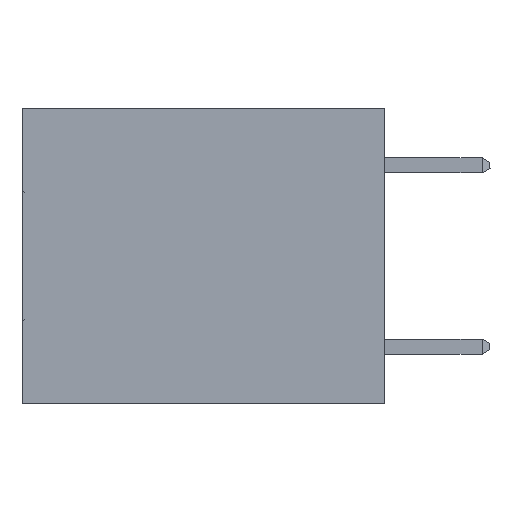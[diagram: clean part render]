
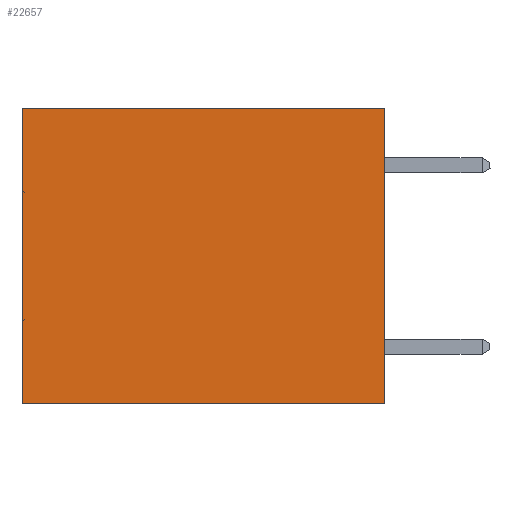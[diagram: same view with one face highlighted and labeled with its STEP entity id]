
A CAD part, left-side view. The second image highlights one B-rep face of the part: STEP entity #22657.
In plain terms, the highlighted planar face has unit normal (-1, 0, 0).
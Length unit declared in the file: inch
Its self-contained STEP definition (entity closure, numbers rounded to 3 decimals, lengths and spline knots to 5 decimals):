
#1168 = VERTEX_POINT ( 'NONE', #27667 ) ;
#1474 = ORIENTED_EDGE ( 'NONE', *, *, #30257, .F. ) ;
#2289 = LINE ( 'NONE', #6628, #15596 ) ;
#2454 = VERTEX_POINT ( 'NONE', #10297 ) ;
#2836 = CARTESIAN_POINT ( 'NONE',  ( 0.3165, 0., -0.49 ) ) ;
#3330 = CARTESIAN_POINT ( 'NONE',  ( 0.3165, 0.6, -0.49 ) ) ;
#3703 = CARTESIAN_POINT ( 'NONE',  ( 0.3165, 0., -0.49 ) ) ;
#4158 = DIRECTION ( 'NONE',  ( 0., 0., -1. ) ) ;
#5411 = EDGE_LOOP ( 'NONE', ( #5615, #31204, #1474, #15413 ) ) ;
#5615 = ORIENTED_EDGE ( 'NONE', *, *, #16350, .T. ) ;
#6628 = CARTESIAN_POINT ( 'NONE',  ( 0.3165, 0., -0.49 ) ) ;
#10297 = CARTESIAN_POINT ( 'NONE',  ( 0.3165, 0.6, -0.49 ) ) ;
#12359 = CARTESIAN_POINT ( 'NONE',  ( 0.3165, 0., 0. ) ) ;
#13540 = AXIS2_PLACEMENT_3D ( 'NONE', #3703, #14599, #28306 ) ;
#13946 = VERTEX_POINT ( 'NONE', #24850 ) ;
#14599 = DIRECTION ( 'NONE',  ( 1., 0., 0. ) ) ;
#15327 = VERTEX_POINT ( 'NONE', #22479 ) ;
#15413 = ORIENTED_EDGE ( 'NONE', *, *, #15735, .T. ) ;
#15596 = VECTOR ( 'NONE', #20298, 39.37008 ) ;
#15735 = EDGE_CURVE ( 'NONE', #1168, #13946, #17672, .T. ) ;
#16350 = EDGE_CURVE ( 'NONE', #13946, #2454, #23231, .T. ) ;
#17672 = LINE ( 'NONE', #12359, #35320 ) ;
#18917 = LINE ( 'NONE', #2836, #31012 ) ;
#20298 = DIRECTION ( 'NONE',  ( 0., 1., 0. ) ) ;
#20661 = DIRECTION ( 'NONE',  ( 0., 1., 0. ) ) ;
#22479 = CARTESIAN_POINT ( 'NONE',  ( 0.3165, 0., -0.49 ) ) ;
#22657 = ADVANCED_FACE ( 'NONE', ( #30470 ), #22761, .F. ) ;
#22761 = PLANE ( 'NONE',  #13540 ) ;
#23231 = LINE ( 'NONE', #3330, #31427 ) ;
#24850 = CARTESIAN_POINT ( 'NONE',  ( 0.3165, 0.6, 0. ) ) ;
#27667 = CARTESIAN_POINT ( 'NONE',  ( 0.3165, 0., 0. ) ) ;
#28306 = DIRECTION ( 'NONE',  ( 0., 0., -1. ) ) ;
#30257 = EDGE_CURVE ( 'NONE', #1168, #15327, #18917, .T. ) ;
#30470 = FACE_OUTER_BOUND ( 'NONE', #5411, .T. ) ;
#30965 = DIRECTION ( 'NONE',  ( 0., 0., -1. ) ) ;
#31012 = VECTOR ( 'NONE', #4158, 39.37008 ) ;
#31204 = ORIENTED_EDGE ( 'NONE', *, *, #35164, .F. ) ;
#31427 = VECTOR ( 'NONE', #30965, 39.37008 ) ;
#35164 = EDGE_CURVE ( 'NONE', #15327, #2454, #2289, .T. ) ;
#35320 = VECTOR ( 'NONE', #20661, 39.37008 ) ;
